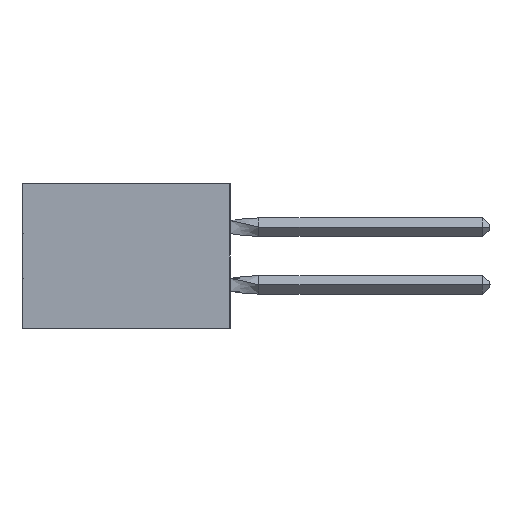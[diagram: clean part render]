
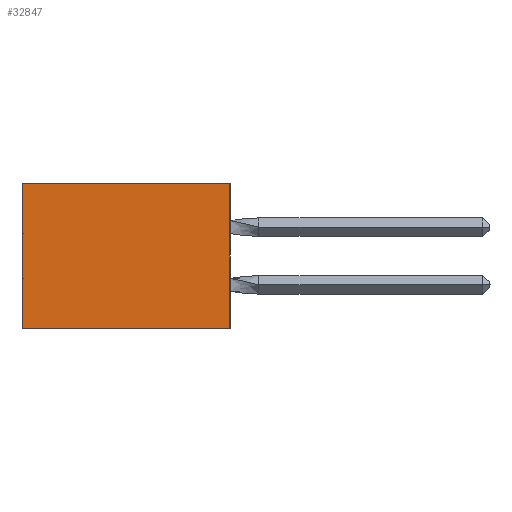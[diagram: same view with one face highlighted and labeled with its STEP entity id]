
A CAD part, left-side view. The second image highlights one B-rep face of the part: STEP entity #32847.
In plain terms, the highlighted planar face has unit normal (-1, 0, 0).
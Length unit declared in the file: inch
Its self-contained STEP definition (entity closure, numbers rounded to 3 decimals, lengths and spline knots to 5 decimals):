
#2215 = CARTESIAN_POINT ( 'NONE',  ( 0.305, 0.72, -0.5 ) ) ;
#2535 = CARTESIAN_POINT ( 'NONE',  ( 0.305, 0., 0. ) ) ;
#3101 = VERTEX_POINT ( 'NONE', #39092 ) ;
#3186 = LINE ( 'NONE', #35778, #26013 ) ;
#4029 = VERTEX_POINT ( 'NONE', #2535 ) ;
#5505 = EDGE_CURVE ( 'NONE', #4029, #3101, #3186, .T. ) ;
#6229 = ORIENTED_EDGE ( 'NONE', *, *, #30393, .F. ) ;
#11441 = VECTOR ( 'NONE', #35145, 39.37008 ) ;
#16696 = EDGE_CURVE ( 'NONE', #3101, #21824, #36102, .T. ) ;
#17661 = VERTEX_POINT ( 'NONE', #44882 ) ;
#17765 = ORIENTED_EDGE ( 'NONE', *, *, #28233, .F. ) ;
#19043 = VECTOR ( 'NONE', #26064, 39.37008 ) ;
#21147 = PLANE ( 'NONE',  #32264 ) ;
#21824 = VERTEX_POINT ( 'NONE', #2215 ) ;
#23789 = LINE ( 'NONE', #48428, #19043 ) ;
#24944 = DIRECTION ( 'NONE',  ( 1., 0., 0. ) ) ;
#26013 = VECTOR ( 'NONE', #43312, 39.37008 ) ;
#26064 = DIRECTION ( 'NONE',  ( 0., 1., 0. ) ) ;
#28190 = FACE_OUTER_BOUND ( 'NONE', #30812, .T. ) ;
#28233 = EDGE_CURVE ( 'NONE', #4029, #17661, #37121, .T. ) ;
#29653 = ORIENTED_EDGE ( 'NONE', *, *, #5505, .T. ) ;
#30393 = EDGE_CURVE ( 'NONE', #17661, #21824, #23789, .T. ) ;
#30812 = EDGE_LOOP ( 'NONE', ( #43025, #6229, #17765, #29653 ) ) ;
#31454 = CARTESIAN_POINT ( 'NONE',  ( 0.305, 0., -0.5 ) ) ;
#32264 = AXIS2_PLACEMENT_3D ( 'NONE', #47298, #24944, #32432 ) ;
#32432 = DIRECTION ( 'NONE',  ( 0., 0., -1. ) ) ;
#32847 = ADVANCED_FACE ( 'NONE', ( #28190 ), #21147, .F. ) ;
#35145 = DIRECTION ( 'NONE',  ( 0., 0., -1. ) ) ;
#35778 = CARTESIAN_POINT ( 'NONE',  ( 0.305, 0., 0. ) ) ;
#36102 = LINE ( 'NONE', #46696, #11441 ) ;
#37121 = LINE ( 'NONE', #31454, #40614 ) ;
#39092 = CARTESIAN_POINT ( 'NONE',  ( 0.305, 0.72, 0. ) ) ;
#39168 = DIRECTION ( 'NONE',  ( 0., 0., -1. ) ) ;
#40614 = VECTOR ( 'NONE', #39168, 39.37008 ) ;
#43025 = ORIENTED_EDGE ( 'NONE', *, *, #16696, .T. ) ;
#43312 = DIRECTION ( 'NONE',  ( 0., 1., 0. ) ) ;
#44882 = CARTESIAN_POINT ( 'NONE',  ( 0.305, 0., -0.5 ) ) ;
#46696 = CARTESIAN_POINT ( 'NONE',  ( 0.305, 0.72, -0.5 ) ) ;
#47298 = CARTESIAN_POINT ( 'NONE',  ( 0.305, 0., -0.5 ) ) ;
#48428 = CARTESIAN_POINT ( 'NONE',  ( 0.305, 0., -0.5 ) ) ;
